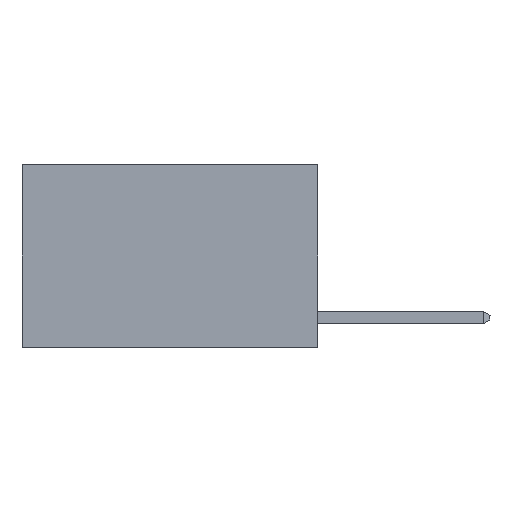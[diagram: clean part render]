
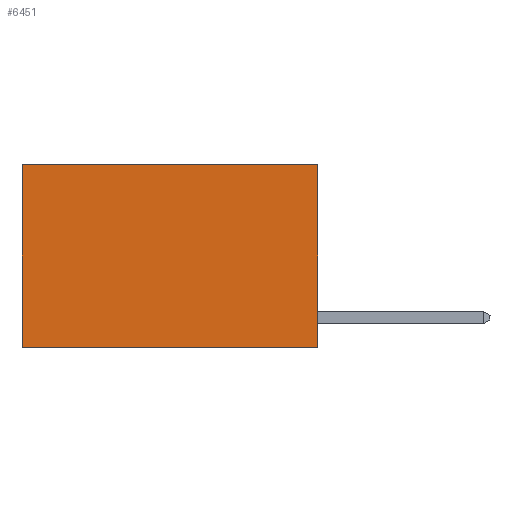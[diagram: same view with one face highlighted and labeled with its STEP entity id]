
A CAD part, left-side view. The second image highlights one B-rep face of the part: STEP entity #6451.
In plain terms, the highlighted planar face has unit normal (-1, 0, 0).
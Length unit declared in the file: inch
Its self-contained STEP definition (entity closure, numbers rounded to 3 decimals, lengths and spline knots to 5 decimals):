
#595 = VECTOR ( 'NONE', #12995, 39.37008 ) ;
#1003 = ORIENTED_EDGE ( 'NONE', *, *, #11963, .T. ) ;
#1843 = VECTOR ( 'NONE', #10020, 39.37008 ) ;
#2846 = CARTESIAN_POINT ( 'NONE',  ( 0.2625, 0., 0. ) ) ;
#3825 = LINE ( 'NONE', #22740, #1843 ) ;
#3845 = FACE_OUTER_BOUND ( 'NONE', #17111, .T. ) ;
#4516 = LINE ( 'NONE', #15065, #595 ) ;
#5650 = VERTEX_POINT ( 'NONE', #23333 ) ;
#6451 = ADVANCED_FACE ( 'NONE', ( #3845 ), #25567, .F. ) ;
#6556 = DIRECTION ( 'NONE',  ( 1., 0., 0. ) ) ;
#6836 = ORIENTED_EDGE ( 'NONE', *, *, #10937, .F. ) ;
#6844 = VECTOR ( 'NONE', #16133, 39.37008 ) ;
#7623 = CARTESIAN_POINT ( 'NONE',  ( 0.2625, 0., -0.37 ) ) ;
#9379 = VECTOR ( 'NONE', #9860, 39.37008 ) ;
#9593 = CARTESIAN_POINT ( 'NONE',  ( 0.2625, 0.6, -0.37 ) ) ;
#9860 = DIRECTION ( 'NONE',  ( 0., 1., 0. ) ) ;
#10020 = DIRECTION ( 'NONE',  ( 0., 0., -1. ) ) ;
#10312 = CARTESIAN_POINT ( 'NONE',  ( 0.2625, 0.6, 0. ) ) ;
#10338 = CARTESIAN_POINT ( 'NONE',  ( 0.2625, 0., 0. ) ) ;
#10937 = EDGE_CURVE ( 'NONE', #26971, #5650, #4516, .T. ) ;
#11963 = EDGE_CURVE ( 'NONE', #25638, #24191, #3825, .T. ) ;
#12630 = AXIS2_PLACEMENT_3D ( 'NONE', #21046, #6556, #12926 ) ;
#12926 = DIRECTION ( 'NONE',  ( 0., 0., -1. ) ) ;
#12995 = DIRECTION ( 'NONE',  ( 0., 0., -1. ) ) ;
#13251 = ORIENTED_EDGE ( 'NONE', *, *, #14736, .F. ) ;
#13431 = EDGE_CURVE ( 'NONE', #26971, #25638, #25170, .T. ) ;
#14736 = EDGE_CURVE ( 'NONE', #5650, #24191, #18062, .T. ) ;
#15065 = CARTESIAN_POINT ( 'NONE',  ( 0.2625, 0., 0. ) ) ;
#16133 = DIRECTION ( 'NONE',  ( 0., 1., 0. ) ) ;
#17111 = EDGE_LOOP ( 'NONE', ( #1003, #13251, #6836, #22553 ) ) ;
#18062 = LINE ( 'NONE', #7623, #6844 ) ;
#21046 = CARTESIAN_POINT ( 'NONE',  ( 0.2625, 0., 0. ) ) ;
#22553 = ORIENTED_EDGE ( 'NONE', *, *, #13431, .T. ) ;
#22740 = CARTESIAN_POINT ( 'NONE',  ( 0.2625, 0.6, 0. ) ) ;
#23333 = CARTESIAN_POINT ( 'NONE',  ( 0.2625, 0., -0.37 ) ) ;
#24191 = VERTEX_POINT ( 'NONE', #9593 ) ;
#25170 = LINE ( 'NONE', #2846, #9379 ) ;
#25567 = PLANE ( 'NONE',  #12630 ) ;
#25638 = VERTEX_POINT ( 'NONE', #10312 ) ;
#26971 = VERTEX_POINT ( 'NONE', #10338 ) ;
